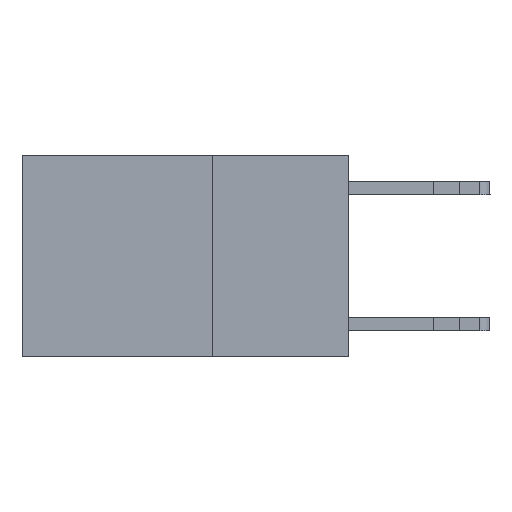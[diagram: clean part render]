
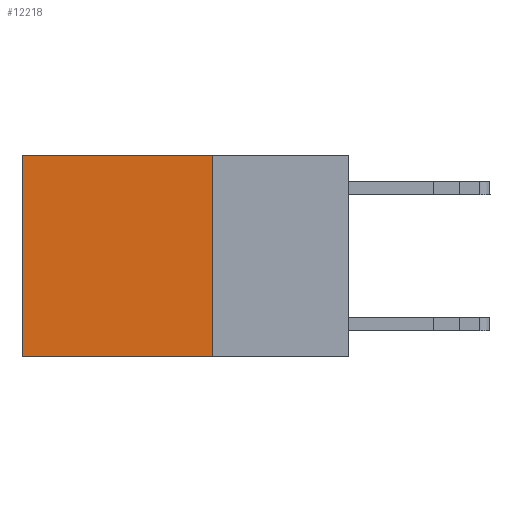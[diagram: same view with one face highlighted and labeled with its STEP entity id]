
A CAD part, left-side view. The second image highlights one B-rep face of the part: STEP entity #12218.
In plain terms, the highlighted planar face has unit normal (-1, 0, 0).
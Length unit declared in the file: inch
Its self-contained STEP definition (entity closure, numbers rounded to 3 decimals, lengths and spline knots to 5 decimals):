
#174 = DIRECTION ( 'NONE',  ( 1., 0., 0. ) ) ;
#1154 = EDGE_CURVE ( 'NONE', #11430, #2632, #6597, .T. ) ;
#2021 = CARTESIAN_POINT ( 'NONE',  ( 0.2625, 0.6, 0. ) ) ;
#2049 = VERTEX_POINT ( 'NONE', #14868 ) ;
#2053 = EDGE_CURVE ( 'NONE', #4384, #2049, #9871, .T. ) ;
#2300 = ORIENTED_EDGE ( 'NONE', *, *, #7238, .T. ) ;
#2632 = VERTEX_POINT ( 'NONE', #7207 ) ;
#4184 = DIRECTION ( 'NONE',  ( 0., 0., -1. ) ) ;
#4384 = VERTEX_POINT ( 'NONE', #10881 ) ;
#4826 = ORIENTED_EDGE ( 'NONE', *, *, #2053, .T. ) ;
#5820 = EDGE_LOOP ( 'NONE', ( #2300, #10258, #15281, #4826 ) ) ;
#5920 = CARTESIAN_POINT ( 'NONE',  ( 0.2625, 0.25, -0.37 ) ) ;
#6115 = VECTOR ( 'NONE', #16224, 39.37008 ) ;
#6324 = DIRECTION ( 'NONE',  ( 0., 0., -1. ) ) ;
#6597 = LINE ( 'NONE', #5920, #8392 ) ;
#7207 = CARTESIAN_POINT ( 'NONE',  ( 0.2625, 0.6, -0.37 ) ) ;
#7238 = EDGE_CURVE ( 'NONE', #2049, #2632, #13325, .T. ) ;
#7379 = PLANE ( 'NONE',  #8800 ) ;
#8392 = VECTOR ( 'NONE', #15649, 39.37008 ) ;
#8800 = AXIS2_PLACEMENT_3D ( 'NONE', #17049, #174, #10186 ) ;
#8933 = VECTOR ( 'NONE', #4184, 39.37008 ) ;
#8988 = EDGE_CURVE ( 'NONE', #4384, #11430, #9379, .T. ) ;
#9357 = FACE_OUTER_BOUND ( 'NONE', #5820, .T. ) ;
#9379 = LINE ( 'NONE', #15419, #8933 ) ;
#9871 = LINE ( 'NONE', #12122, #6115 ) ;
#10186 = DIRECTION ( 'NONE',  ( 0., 0., -1. ) ) ;
#10258 = ORIENTED_EDGE ( 'NONE', *, *, #1154, .F. ) ;
#10881 = CARTESIAN_POINT ( 'NONE',  ( 0.2625, 0.25, 0. ) ) ;
#10948 = CARTESIAN_POINT ( 'NONE',  ( 0.2625, 0.25, -0.37 ) ) ;
#11430 = VERTEX_POINT ( 'NONE', #10948 ) ;
#12122 = CARTESIAN_POINT ( 'NONE',  ( 0.2625, 0.25, 0. ) ) ;
#12218 = ADVANCED_FACE ( 'NONE', ( #9357 ), #7379, .F. ) ;
#13325 = LINE ( 'NONE', #2021, #16955 ) ;
#14868 = CARTESIAN_POINT ( 'NONE',  ( 0.2625, 0.6, 0. ) ) ;
#15281 = ORIENTED_EDGE ( 'NONE', *, *, #8988, .F. ) ;
#15419 = CARTESIAN_POINT ( 'NONE',  ( 0.2625, 0.25, 0. ) ) ;
#15649 = DIRECTION ( 'NONE',  ( 0., 1., 0. ) ) ;
#16224 = DIRECTION ( 'NONE',  ( 0., 1., 0. ) ) ;
#16955 = VECTOR ( 'NONE', #6324, 39.37008 ) ;
#17049 = CARTESIAN_POINT ( 'NONE',  ( 0.2625, 0.25, 0. ) ) ;
